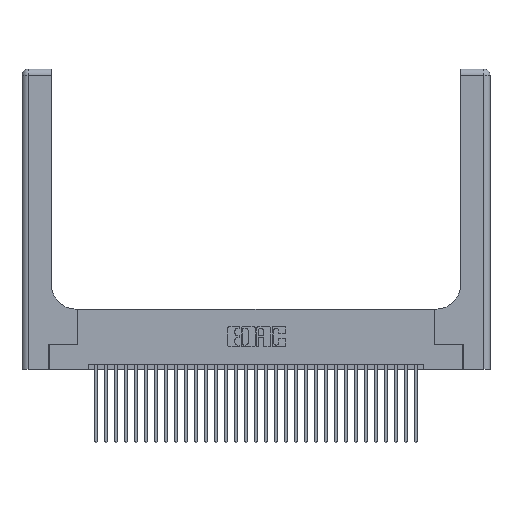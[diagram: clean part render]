
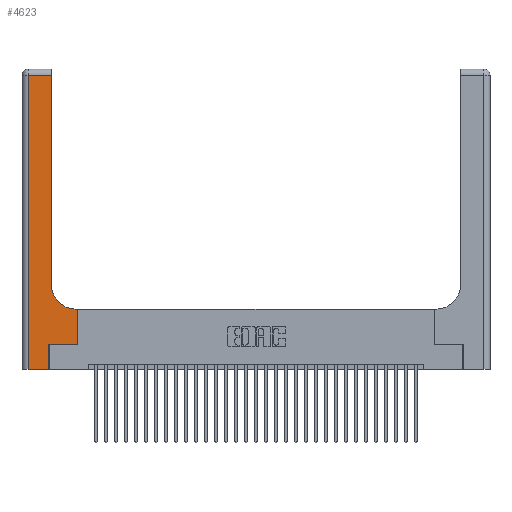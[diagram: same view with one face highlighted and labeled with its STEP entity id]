
A CAD part, top view. The second image highlights one B-rep face of the part: STEP entity #4623.
In plain terms, the highlighted planar face has unit normal (0, 0, 1).
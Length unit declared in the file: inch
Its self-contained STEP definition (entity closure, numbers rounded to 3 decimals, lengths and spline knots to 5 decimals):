
#305 = EDGE_LOOP ( 'NONE', ( #2976, #23705, #29163, #4171, #5738, #21398, #16339, #27673, #29222 ) ) ;
#388 = EDGE_CURVE ( 'NONE', #2758, #9902, #32308, .T. ) ;
#574 = DIRECTION ( 'NONE',  ( 0., -1., 0. ) ) ;
#848 = DIRECTION ( 'NONE',  ( 1., 0., 0. ) ) ;
#1768 = VERTEX_POINT ( 'NONE', #25996 ) ;
#1905 = LINE ( 'NONE', #5229, #21106 ) ;
#2758 = VERTEX_POINT ( 'NONE', #27122 ) ;
#2976 = ORIENTED_EDGE ( 'NONE', *, *, #21743, .T. ) ;
#3307 = CARTESIAN_POINT ( 'NONE',  ( 0.2915, 2.94, 0.37 ) ) ;
#4171 = ORIENTED_EDGE ( 'NONE', *, *, #10799, .T. ) ;
#4623 = ADVANCED_FACE ( 'NONE', ( #12487 ), #6724, .F. ) ;
#5229 = CARTESIAN_POINT ( 'NONE',  ( 0.269, 0., 0.37 ) ) ;
#5738 = ORIENTED_EDGE ( 'NONE', *, *, #14546, .T. ) ;
#6724 = PLANE ( 'NONE',  #27319 ) ;
#7594 = VECTOR ( 'NONE', #9746, 39.37008 ) ;
#8053 = EDGE_CURVE ( 'NONE', #31677, #12988, #21634, .T. ) ;
#8199 = EDGE_CURVE ( 'NONE', #16836, #31677, #24730, .T. ) ;
#8298 = VERTEX_POINT ( 'NONE', #31331 ) ;
#9265 = DIRECTION ( 'NONE',  ( -1., 0., 0. ) ) ;
#9746 = DIRECTION ( 'NONE',  ( -1., 0., 0. ) ) ;
#9902 = VERTEX_POINT ( 'NONE', #32231 ) ;
#10142 = CARTESIAN_POINT ( 'NONE',  ( 0.2915, 3., 0.37 ) ) ;
#10799 = EDGE_CURVE ( 'NONE', #12988, #12815, #21749, .T. ) ;
#11121 = CARTESIAN_POINT ( 'NONE',  ( 0.5415, 0.85, 0.37 ) ) ;
#11369 = AXIS2_PLACEMENT_3D ( 'NONE', #11121, #28553, #13621 ) ;
#12487 = FACE_OUTER_BOUND ( 'NONE', #305, .T. ) ;
#12815 = VERTEX_POINT ( 'NONE', #20873 ) ;
#12988 = VERTEX_POINT ( 'NONE', #21405 ) ;
#13619 = CARTESIAN_POINT ( 'NONE',  ( 0., 2.94, 0.37 ) ) ;
#13621 = DIRECTION ( 'NONE',  ( 1., 0., 0. ) ) ;
#14546 = EDGE_CURVE ( 'NONE', #12815, #1768, #1905, .T. ) ;
#15115 = VECTOR ( 'NONE', #848, 39.37008 ) ;
#15160 = DIRECTION ( 'NONE',  ( 0., 1., 0. ) ) ;
#15592 = DIRECTION ( 'NONE',  ( 1., 0., 0. ) ) ;
#16148 = DIRECTION ( 'NONE',  ( -1., 0., 0. ) ) ;
#16339 = ORIENTED_EDGE ( 'NONE', *, *, #26785, .T. ) ;
#16423 = VECTOR ( 'NONE', #22888, 39.37008 ) ;
#16836 = VERTEX_POINT ( 'NONE', #3307 ) ;
#17318 = VERTEX_POINT ( 'NONE', #19908 ) ;
#18014 = CARTESIAN_POINT ( 'NONE',  ( 0.06, 3., 0.37 ) ) ;
#18104 = VECTOR ( 'NONE', #16148, 39.37008 ) ;
#18281 = CARTESIAN_POINT ( 'NONE',  ( 0.269, 0.25, 0.37 ) ) ;
#19152 = CARTESIAN_POINT ( 'NONE',  ( 0.06, 2.94, 0.37 ) ) ;
#19908 = CARTESIAN_POINT ( 'NONE',  ( 0.5585, 0.25, 0.37 ) ) ;
#20159 = CARTESIAN_POINT ( 'NONE',  ( 0.5585, 0.25, 0.37 ) ) ;
#20218 = DIRECTION ( 'NONE',  ( 0., 1., 0. ) ) ;
#20342 = VECTOR ( 'NONE', #15160, 39.37008 ) ;
#20860 = VECTOR ( 'NONE', #574, 39.37008 ) ;
#20873 = CARTESIAN_POINT ( 'NONE',  ( 0.269, 0., 0.37 ) ) ;
#21074 = EDGE_CURVE ( 'NONE', #8298, #2758, #21550, .T. ) ;
#21106 = VECTOR ( 'NONE', #20218, 39.37008 ) ;
#21123 = LINE ( 'NONE', #10142, #20342 ) ;
#21398 = ORIENTED_EDGE ( 'NONE', *, *, #22681, .T. ) ;
#21405 = CARTESIAN_POINT ( 'NONE',  ( 0.06, 0., 0.37 ) ) ;
#21550 = LINE ( 'NONE', #24803, #7594 ) ;
#21634 = LINE ( 'NONE', #18014, #20860 ) ;
#21710 = CARTESIAN_POINT ( 'NONE',  ( 0., 3., 0.37 ) ) ;
#21743 = EDGE_CURVE ( 'NONE', #9902, #16836, #21123, .T. ) ;
#21749 = LINE ( 'NONE', #28006, #27598 ) ;
#21760 = LINE ( 'NONE', #18281, #15115 ) ;
#22681 = EDGE_CURVE ( 'NONE', #1768, #17318, #21760, .T. ) ;
#22888 = DIRECTION ( 'NONE',  ( 0., 1., 0. ) ) ;
#23053 = LINE ( 'NONE', #20159, #16423 ) ;
#23705 = ORIENTED_EDGE ( 'NONE', *, *, #8199, .T. ) ;
#24216 = DIRECTION ( 'NONE',  ( 0., 0., -1. ) ) ;
#24730 = LINE ( 'NONE', #13619, #18104 ) ;
#24803 = CARTESIAN_POINT ( 'NONE',  ( 0.2915, 0.6, 0.37 ) ) ;
#25996 = CARTESIAN_POINT ( 'NONE',  ( 0.269, 0.25, 0.37 ) ) ;
#26785 = EDGE_CURVE ( 'NONE', #17318, #8298, #23053, .T. ) ;
#27122 = CARTESIAN_POINT ( 'NONE',  ( 0.5415, 0.6, 0.37 ) ) ;
#27319 = AXIS2_PLACEMENT_3D ( 'NONE', #21710, #24216, #9265 ) ;
#27598 = VECTOR ( 'NONE', #15592, 39.37008 ) ;
#27673 = ORIENTED_EDGE ( 'NONE', *, *, #21074, .T. ) ;
#28006 = CARTESIAN_POINT ( 'NONE',  ( 0., 0., 0.37 ) ) ;
#28553 = DIRECTION ( 'NONE',  ( 0., 0., -1. ) ) ;
#29163 = ORIENTED_EDGE ( 'NONE', *, *, #8053, .T. ) ;
#29222 = ORIENTED_EDGE ( 'NONE', *, *, #388, .T. ) ;
#31331 = CARTESIAN_POINT ( 'NONE',  ( 0.5585, 0.6, 0.37 ) ) ;
#31677 = VERTEX_POINT ( 'NONE', #19152 ) ;
#32231 = CARTESIAN_POINT ( 'NONE',  ( 0.2915, 0.85, 0.37 ) ) ;
#32308 = CIRCLE ( 'NONE', #11369, 0.25 ) ;
